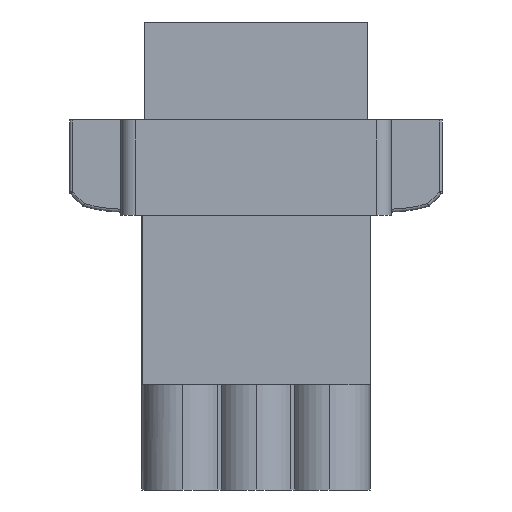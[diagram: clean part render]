
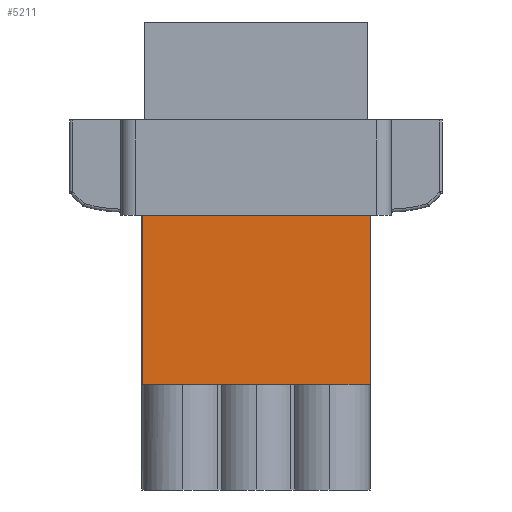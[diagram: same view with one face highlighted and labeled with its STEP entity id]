
A CAD part, front view. The second image highlights one B-rep face of the part: STEP entity #5211.
In plain terms, the highlighted planar face has unit normal (0, -1, 0).
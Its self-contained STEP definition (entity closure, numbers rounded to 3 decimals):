
#44 = LINE ( 'NONE', #9825, #10246 ) ;
#203 = LINE ( 'NONE', #6886, #6224 ) ;
#652 = CARTESIAN_POINT ( 'NONE',  ( -7.775, -0.4, -11.6 ) ) ;
#1053 = ORIENTED_EDGE ( 'NONE', *, *, #7040, .T. ) ;
#1492 = EDGE_CURVE ( 'NONE', #8792, #9534, #203, .T. ) ;
#1513 = DIRECTION ( 'NONE',  ( 0., 1., 0. ) ) ;
#1927 = CARTESIAN_POINT ( 'NONE',  ( -7.775, -0.4, 0. ) ) ;
#2317 = FACE_OUTER_BOUND ( 'NONE', #7741, .T. ) ;
#3227 = CARTESIAN_POINT ( 'NONE',  ( 7.8, -0.4, 0. ) ) ;
#3303 = ORIENTED_EDGE ( 'NONE', *, *, #1492, .F. ) ;
#3920 = CARTESIAN_POINT ( 'NONE',  ( -7.775, -0.4, -11.6 ) ) ;
#4344 = EDGE_CURVE ( 'NONE', #10143, #5318, #7093, .T. ) ;
#4397 = VECTOR ( 'NONE', #8805, 1000. ) ;
#4426 = DIRECTION ( 'NONE',  ( 0., 0., 1. ) ) ;
#4742 = EDGE_CURVE ( 'NONE', #10143, #8792, #7081, .T. ) ;
#5092 = CARTESIAN_POINT ( 'NONE',  ( 7.8, -0.4, -11.6 ) ) ;
#5211 = ADVANCED_FACE ( 'NONE', ( #2317 ), #7979, .F. ) ;
#5318 = VERTEX_POINT ( 'NONE', #3227 ) ;
#5548 = CARTESIAN_POINT ( 'NONE',  ( 7.8, -0.4, -11.6 ) ) ;
#6224 = VECTOR ( 'NONE', #4426, 1000. ) ;
#6886 = CARTESIAN_POINT ( 'NONE',  ( -7.775, -0.4, -11.6 ) ) ;
#7040 = EDGE_CURVE ( 'NONE', #5318, #9534, #44, .T. ) ;
#7081 = LINE ( 'NONE', #9491, #9543 ) ;
#7093 = LINE ( 'NONE', #5548, #4397 ) ;
#7175 = DIRECTION ( 'NONE',  ( 0., 0., 1. ) ) ;
#7741 = EDGE_LOOP ( 'NONE', ( #1053, #3303, #9012, #9706 ) ) ;
#7941 = DIRECTION ( 'NONE',  ( -1., 0., 0. ) ) ;
#7979 = PLANE ( 'NONE',  #10570 ) ;
#8792 = VERTEX_POINT ( 'NONE', #3920 ) ;
#8805 = DIRECTION ( 'NONE',  ( 0., 0., 1. ) ) ;
#9012 = ORIENTED_EDGE ( 'NONE', *, *, #4742, .F. ) ;
#9491 = CARTESIAN_POINT ( 'NONE',  ( -7.775, -0.4, -11.6 ) ) ;
#9534 = VERTEX_POINT ( 'NONE', #1927 ) ;
#9543 = VECTOR ( 'NONE', #7941, 1000. ) ;
#9706 = ORIENTED_EDGE ( 'NONE', *, *, #4344, .T. ) ;
#9825 = CARTESIAN_POINT ( 'NONE',  ( -7.775, -0.4, 0. ) ) ;
#10143 = VERTEX_POINT ( 'NONE', #5092 ) ;
#10246 = VECTOR ( 'NONE', #10403, 1000. ) ;
#10403 = DIRECTION ( 'NONE',  ( -1., 0., 0. ) ) ;
#10570 = AXIS2_PLACEMENT_3D ( 'NONE', #652, #1513, #7175 ) ;
